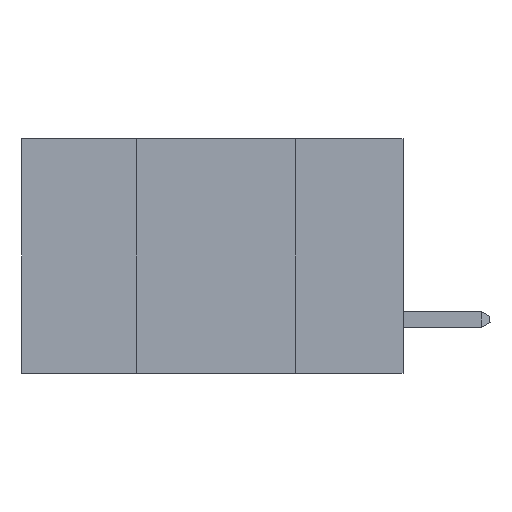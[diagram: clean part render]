
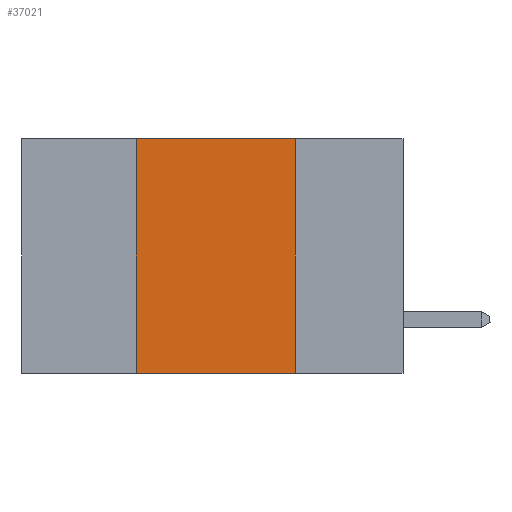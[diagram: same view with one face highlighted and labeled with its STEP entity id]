
A CAD part, left-side view. The second image highlights one B-rep face of the part: STEP entity #37021.
In plain terms, the highlighted planar face has unit normal (-1, 0, 0).
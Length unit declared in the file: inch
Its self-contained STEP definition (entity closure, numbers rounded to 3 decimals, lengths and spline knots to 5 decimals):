
#252 = CARTESIAN_POINT ( 'NONE',  ( 0., 0.17, 0. ) ) ;
#906 = PLANE ( 'NONE',  #34294 ) ;
#1405 = VERTEX_POINT ( 'NONE', #12644 ) ;
#1968 = DIRECTION ( 'NONE',  ( 0., -1., 0. ) ) ;
#3011 = EDGE_CURVE ( 'NONE', #1405, #24940, #42236, .T. ) ;
#7848 = LINE ( 'NONE', #20923, #39921 ) ;
#10615 = VECTOR ( 'NONE', #14205, 39.37008 ) ;
#10623 = CARTESIAN_POINT ( 'NONE',  ( 0., 0.6, 0. ) ) ;
#11799 = CARTESIAN_POINT ( 'NONE',  ( 0., 0.6, -0.37 ) ) ;
#12551 = ORIENTED_EDGE ( 'NONE', *, *, #28029, .F. ) ;
#12644 = CARTESIAN_POINT ( 'NONE',  ( 0., 0.42, -0.37 ) ) ;
#12876 = ORIENTED_EDGE ( 'NONE', *, *, #3011, .F. ) ;
#13328 = VECTOR ( 'NONE', #27538, 39.37008 ) ;
#14205 = DIRECTION ( 'NONE',  ( 0., 0., 1. ) ) ;
#15046 = CARTESIAN_POINT ( 'NONE',  ( 0., 0.42, 0. ) ) ;
#16474 = LINE ( 'NONE', #40413, #13328 ) ;
#19838 = EDGE_CURVE ( 'NONE', #24940, #36293, #7848, .T. ) ;
#20923 = CARTESIAN_POINT ( 'NONE',  ( 0., 0.6, 0. ) ) ;
#22181 = VECTOR ( 'NONE', #1968, 39.37008 ) ;
#24940 = VERTEX_POINT ( 'NONE', #15046 ) ;
#25504 = EDGE_CURVE ( 'NONE', #1405, #40433, #40800, .T. ) ;
#27538 = DIRECTION ( 'NONE',  ( 0., 0., -1. ) ) ;
#28029 = EDGE_CURVE ( 'NONE', #36293, #40433, #16474, .T. ) ;
#29413 = FACE_OUTER_BOUND ( 'NONE', #29864, .T. ) ;
#29864 = EDGE_LOOP ( 'NONE', ( #12551, #39258, #12876, #35348 ) ) ;
#30586 = DIRECTION ( 'NONE',  ( 1., 0., 0. ) ) ;
#31021 = DIRECTION ( 'NONE',  ( 0., 0., -1. ) ) ;
#31210 = DIRECTION ( 'NONE',  ( 0., -1., 0. ) ) ;
#34294 = AXIS2_PLACEMENT_3D ( 'NONE', #10623, #30586, #31021 ) ;
#35348 = ORIENTED_EDGE ( 'NONE', *, *, #25504, .T. ) ;
#36293 = VERTEX_POINT ( 'NONE', #252 ) ;
#37021 = ADVANCED_FACE ( 'NONE', ( #29413 ), #906, .F. ) ;
#39258 = ORIENTED_EDGE ( 'NONE', *, *, #19838, .F. ) ;
#39921 = VECTOR ( 'NONE', #31210, 39.37008 ) ;
#40413 = CARTESIAN_POINT ( 'NONE',  ( 0., 0.17, 0. ) ) ;
#40433 = VERTEX_POINT ( 'NONE', #42041 ) ;
#40800 = LINE ( 'NONE', #11799, #22181 ) ;
#42041 = CARTESIAN_POINT ( 'NONE',  ( 0., 0.17, -0.37 ) ) ;
#42233 = CARTESIAN_POINT ( 'NONE',  ( 0., 0.42, 0. ) ) ;
#42236 = LINE ( 'NONE', #42233, #10615 ) ;
